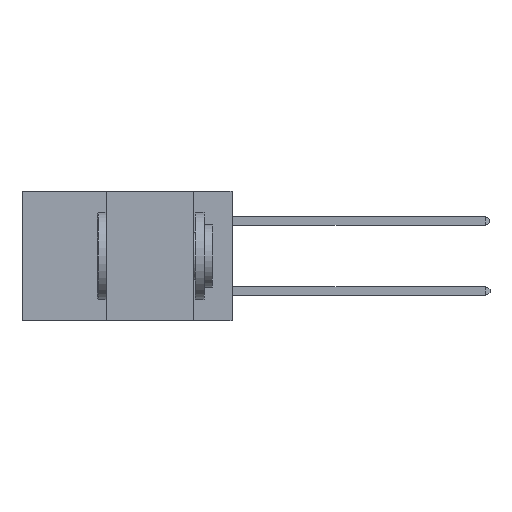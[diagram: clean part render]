
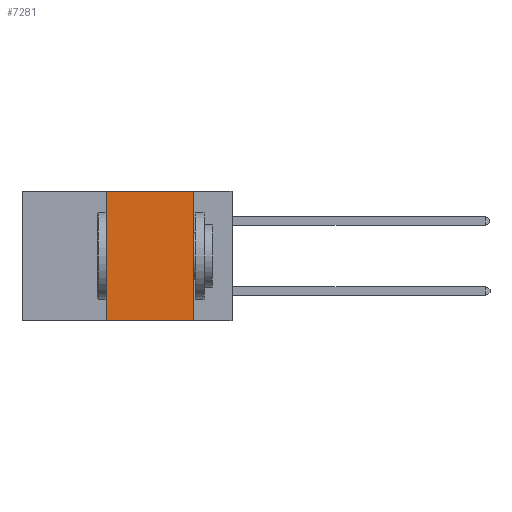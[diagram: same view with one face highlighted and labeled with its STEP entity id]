
A CAD part, left-side view. The second image highlights one B-rep face of the part: STEP entity #7281.
In plain terms, the highlighted planar face has unit normal (-1, 0, 0).
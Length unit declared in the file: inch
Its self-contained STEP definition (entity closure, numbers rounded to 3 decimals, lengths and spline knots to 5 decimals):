
#1384 = DIRECTION ( 'NONE',  ( 1., 0., 0. ) ) ;
#2300 = ORIENTED_EDGE ( 'NONE', *, *, #8498, .F. ) ;
#2420 = VERTEX_POINT ( 'NONE', #4215 ) ;
#2871 = LINE ( 'NONE', #17343, #6468 ) ;
#3511 = VECTOR ( 'NONE', #11842, 39.37008 ) ;
#4215 = CARTESIAN_POINT ( 'NONE',  ( 0., 0.36, 0. ) ) ;
#4472 = LINE ( 'NONE', #5634, #3511 ) ;
#4865 = CARTESIAN_POINT ( 'NONE',  ( 0., 0.11, 0. ) ) ;
#5634 = CARTESIAN_POINT ( 'NONE',  ( 0., 0.6, 0. ) ) ;
#5735 = CARTESIAN_POINT ( 'NONE',  ( 0., 0.36, 0. ) ) ;
#6376 = ORIENTED_EDGE ( 'NONE', *, *, #11112, .F. ) ;
#6468 = VECTOR ( 'NONE', #9678, 39.37008 ) ;
#7281 = ADVANCED_FACE ( 'NONE', ( #12974 ), #18240, .F. ) ;
#7704 = CARTESIAN_POINT ( 'NONE',  ( 0., 0.11, 0. ) ) ;
#7949 = LINE ( 'NONE', #7704, #15195 ) ;
#8498 = EDGE_CURVE ( 'NONE', #2420, #15626, #4472, .T. ) ;
#9153 = AXIS2_PLACEMENT_3D ( 'NONE', #19785, #1384, #12162 ) ;
#9226 = ORIENTED_EDGE ( 'NONE', *, *, #11901, .F. ) ;
#9661 = VECTOR ( 'NONE', #16479, 39.37008 ) ;
#9678 = DIRECTION ( 'NONE',  ( 0., -1., 0. ) ) ;
#10956 = CARTESIAN_POINT ( 'NONE',  ( 0., 0.11, -0.37 ) ) ;
#11112 = EDGE_CURVE ( 'NONE', #14375, #2420, #13318, .T. ) ;
#11662 = EDGE_LOOP ( 'NONE', ( #9226, #2300, #6376, #14087 ) ) ;
#11842 = DIRECTION ( 'NONE',  ( 0., -1., 0. ) ) ;
#11901 = EDGE_CURVE ( 'NONE', #15626, #11981, #7949, .T. ) ;
#11981 = VERTEX_POINT ( 'NONE', #10956 ) ;
#12162 = DIRECTION ( 'NONE',  ( 0., 0., -1. ) ) ;
#12974 = FACE_OUTER_BOUND ( 'NONE', #11662, .T. ) ;
#13318 = LINE ( 'NONE', #5735, #9661 ) ;
#13833 = EDGE_CURVE ( 'NONE', #14375, #11981, #2871, .T. ) ;
#14087 = ORIENTED_EDGE ( 'NONE', *, *, #13833, .T. ) ;
#14375 = VERTEX_POINT ( 'NONE', #18668 ) ;
#15195 = VECTOR ( 'NONE', #18473, 39.37008 ) ;
#15626 = VERTEX_POINT ( 'NONE', #4865 ) ;
#16479 = DIRECTION ( 'NONE',  ( 0., 0., 1. ) ) ;
#17343 = CARTESIAN_POINT ( 'NONE',  ( 0., 0.6, -0.37 ) ) ;
#18240 = PLANE ( 'NONE',  #9153 ) ;
#18473 = DIRECTION ( 'NONE',  ( 0., 0., -1. ) ) ;
#18668 = CARTESIAN_POINT ( 'NONE',  ( 0., 0.36, -0.37 ) ) ;
#19785 = CARTESIAN_POINT ( 'NONE',  ( 0., 0.6, 0. ) ) ;
